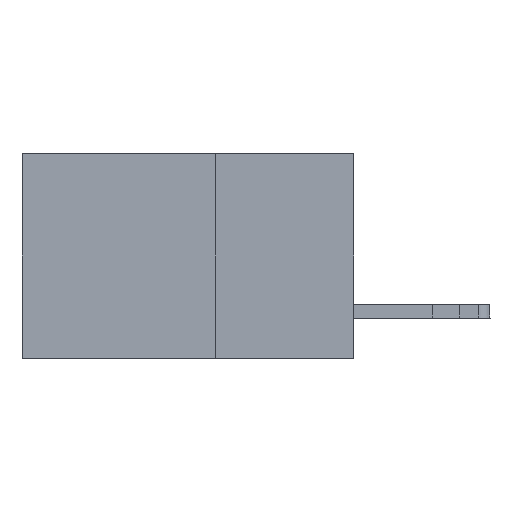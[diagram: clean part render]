
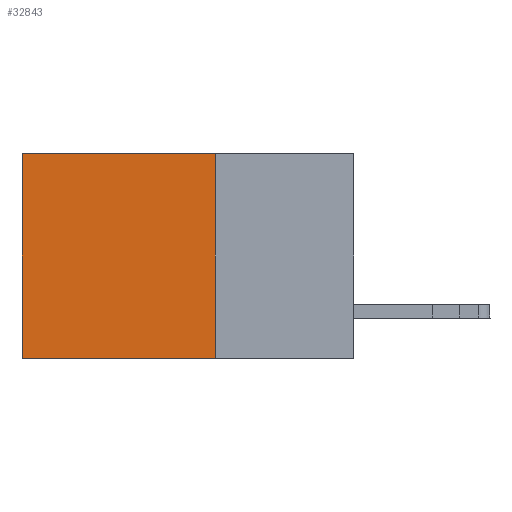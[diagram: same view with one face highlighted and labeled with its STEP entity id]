
A CAD part, left-side view. The second image highlights one B-rep face of the part: STEP entity #32843.
In plain terms, the highlighted planar face has unit normal (-1, 0, 0).
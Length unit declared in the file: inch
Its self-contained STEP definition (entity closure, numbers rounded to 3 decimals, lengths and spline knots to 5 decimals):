
#11 = DIRECTION ( 'NONE',  ( 0., 0., -1. ) ) ;
#278 = CARTESIAN_POINT ( 'NONE',  ( 0.2875, 0.25, 0. ) ) ;
#1149 = DIRECTION ( 'NONE',  ( 0., 0., -1. ) ) ;
#4379 = DIRECTION ( 'NONE',  ( 0., 1., 0. ) ) ;
#4867 = DIRECTION ( 'NONE',  ( 0., 1., 0. ) ) ;
#5362 = CARTESIAN_POINT ( 'NONE',  ( 0.2875, 0.25, -0.37 ) ) ;
#6397 = LINE ( 'NONE', #15970, #24891 ) ;
#6672 = VERTEX_POINT ( 'NONE', #15476 ) ;
#11321 = ORIENTED_EDGE ( 'NONE', *, *, #13833, .T. ) ;
#12387 = VECTOR ( 'NONE', #4867, 39.37008 ) ;
#12519 = ORIENTED_EDGE ( 'NONE', *, *, #24457, .T. ) ;
#13530 = DIRECTION ( 'NONE',  ( 0., 0., -1. ) ) ;
#13833 = EDGE_CURVE ( 'NONE', #19065, #29648, #6397, .T. ) ;
#14031 = PLANE ( 'NONE',  #23173 ) ;
#14143 = LINE ( 'NONE', #5362, #12387 ) ;
#15476 = CARTESIAN_POINT ( 'NONE',  ( 0.2875, 0.25, -0.37 ) ) ;
#15970 = CARTESIAN_POINT ( 'NONE',  ( 0.2875, 0.25, 0. ) ) ;
#16161 = CARTESIAN_POINT ( 'NONE',  ( 0.2875, 0.6, -0.37 ) ) ;
#16840 = DIRECTION ( 'NONE',  ( 1., 0., 0. ) ) ;
#18118 = CARTESIAN_POINT ( 'NONE',  ( 0.2875, 0.25, 0. ) ) ;
#18539 = EDGE_CURVE ( 'NONE', #19065, #6672, #21911, .T. ) ;
#18947 = EDGE_LOOP ( 'NONE', ( #12519, #32690, #22042, #11321 ) ) ;
#19065 = VERTEX_POINT ( 'NONE', #18118 ) ;
#19077 = CARTESIAN_POINT ( 'NONE',  ( 0.2875, 0.6, 0. ) ) ;
#21068 = EDGE_CURVE ( 'NONE', #6672, #27773, #14143, .T. ) ;
#21911 = LINE ( 'NONE', #278, #25399 ) ;
#22042 = ORIENTED_EDGE ( 'NONE', *, *, #18539, .F. ) ;
#22259 = CARTESIAN_POINT ( 'NONE',  ( 0.2875, 0.6, 0. ) ) ;
#22805 = FACE_OUTER_BOUND ( 'NONE', #18947, .T. ) ;
#23173 = AXIS2_PLACEMENT_3D ( 'NONE', #33723, #16840, #11 ) ;
#24457 = EDGE_CURVE ( 'NONE', #29648, #27773, #29743, .T. ) ;
#24891 = VECTOR ( 'NONE', #4379, 39.37008 ) ;
#25399 = VECTOR ( 'NONE', #1149, 39.37008 ) ;
#27773 = VERTEX_POINT ( 'NONE', #16161 ) ;
#29648 = VERTEX_POINT ( 'NONE', #22259 ) ;
#29743 = LINE ( 'NONE', #19077, #35437 ) ;
#32690 = ORIENTED_EDGE ( 'NONE', *, *, #21068, .F. ) ;
#32843 = ADVANCED_FACE ( 'NONE', ( #22805 ), #14031, .F. ) ;
#33723 = CARTESIAN_POINT ( 'NONE',  ( 0.2875, 0.25, 0. ) ) ;
#35437 = VECTOR ( 'NONE', #13530, 39.37008 ) ;
